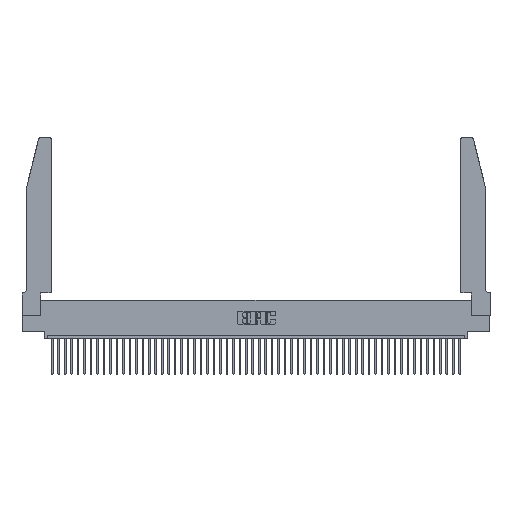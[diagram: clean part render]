
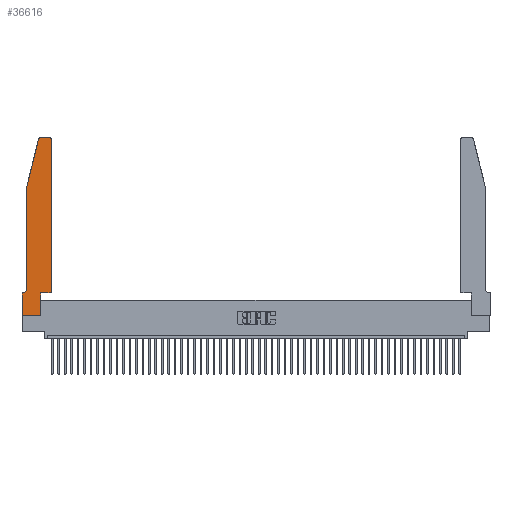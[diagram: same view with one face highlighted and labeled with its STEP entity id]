
A CAD part, top view. The second image highlights one B-rep face of the part: STEP entity #36616.
In plain terms, the highlighted planar face has unit normal (0, 0, 1).
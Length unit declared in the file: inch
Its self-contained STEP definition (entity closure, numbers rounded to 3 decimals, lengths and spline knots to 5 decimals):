
#546 = VECTOR ( 'NONE', #32866, 39.37008 ) ;
#928 = DIRECTION ( 'NONE',  ( 1., 0., 0. ) ) ;
#1456 = ORIENTED_EDGE ( 'NONE', *, *, #26415, .T. ) ;
#2558 = VERTEX_POINT ( 'NONE', #14440 ) ;
#3443 = VERTEX_POINT ( 'NONE', #38005 ) ;
#3659 = VERTEX_POINT ( 'NONE', #14389 ) ;
#3855 = EDGE_CURVE ( 'NONE', #31584, #44310, #7764, .T. ) ;
#4008 = VERTEX_POINT ( 'NONE', #12198 ) ;
#4090 = DIRECTION ( 'NONE',  ( 1., 0., 0. ) ) ;
#5815 = CARTESIAN_POINT ( 'NONE',  ( 0.2865, 0.35, 0.37 ) ) ;
#6371 = DIRECTION ( 'NONE',  ( 0., 0., 1. ) ) ;
#7077 = VERTEX_POINT ( 'NONE', #15256 ) ;
#7407 = VERTEX_POINT ( 'NONE', #23705 ) ;
#7764 = LINE ( 'NONE', #5815, #47663 ) ;
#8116 = EDGE_CURVE ( 'NONE', #3443, #46288, #13813, .T. ) ;
#8571 = CARTESIAN_POINT ( 'NONE',  ( 0.0755, 2., 0.37 ) ) ;
#8710 = DIRECTION ( 'NONE',  ( -1., 0., 0. ) ) ;
#8753 = PLANE ( 'NONE',  #46089 ) ;
#8880 = CARTESIAN_POINT ( 'NONE',  ( 0.0755, 0.35, 0.37 ) ) ;
#9929 = CARTESIAN_POINT ( 'NONE',  ( 0.284, 2.72, 0.37 ) ) ;
#10251 = AXIS2_PLACEMENT_3D ( 'NONE', #9929, #6371, #37412 ) ;
#11137 = EDGE_CURVE ( 'NONE', #2558, #7077, #17133, .T. ) ;
#11425 = EDGE_CURVE ( 'NONE', #7407, #22206, #19561, .T. ) ;
#12198 = CARTESIAN_POINT ( 'NONE',  ( 0.0055, 0.35, 0.37 ) ) ;
#12435 = CARTESIAN_POINT ( 'NONE',  ( 0., 0.35, 0.37 ) ) ;
#13041 = ORIENTED_EDGE ( 'NONE', *, *, #32756, .T. ) ;
#13813 = LINE ( 'NONE', #17291, #546 ) ;
#14202 = LINE ( 'NONE', #15179, #27502 ) ;
#14389 = CARTESIAN_POINT ( 'NONE',  ( 0.0755, 0.42, 0.37 ) ) ;
#14440 = CARTESIAN_POINT ( 'NONE',  ( 0.284, 2.75, 0.37 ) ) ;
#14837 = VECTOR ( 'NONE', #25007, 39.37008 ) ;
#14989 = LINE ( 'NONE', #8880, #25309 ) ;
#15179 = CARTESIAN_POINT ( 'NONE',  ( 0., 0., 0.37 ) ) ;
#15256 = CARTESIAN_POINT ( 'NONE',  ( 0.25487, 2.72718, 0.37 ) ) ;
#15302 = EDGE_CURVE ( 'NONE', #37800, #7407, #28854, .T. ) ;
#15967 = EDGE_CURVE ( 'NONE', #22206, #2558, #49955, .T. ) ;
#16433 = ORIENTED_EDGE ( 'NONE', *, *, #26917, .T. ) ;
#17133 = CIRCLE ( 'NONE', #10251, 0.03 ) ;
#17291 = CARTESIAN_POINT ( 'NONE',  ( 0., 0., 0.37 ) ) ;
#17758 = DIRECTION ( 'NONE',  ( 0., 1., 0. ) ) ;
#17773 = DIRECTION ( 'NONE',  ( 0., 1., 0. ) ) ;
#17872 = CARTESIAN_POINT ( 'NONE',  ( 0.2605, 2.75, 0.37 ) ) ;
#17987 = VECTOR ( 'NONE', #27104, 39.37008 ) ;
#19561 = CIRCLE ( 'NONE', #27385, 0.03 ) ;
#20211 = DIRECTION ( 'NONE',  ( 0., 0., 1. ) ) ;
#21271 = ORIENTED_EDGE ( 'NONE', *, *, #8116, .T. ) ;
#22206 = VERTEX_POINT ( 'NONE', #24424 ) ;
#22641 = DIRECTION ( 'NONE',  ( 1., 0., 0. ) ) ;
#22766 = ORIENTED_EDGE ( 'NONE', *, *, #11137, .T. ) ;
#23705 = CARTESIAN_POINT ( 'NONE',  ( 0.4505, 2.72, 0.37 ) ) ;
#24014 = VERTEX_POINT ( 'NONE', #43203 ) ;
#24424 = CARTESIAN_POINT ( 'NONE',  ( 0.4205, 2.75, 0.37 ) ) ;
#25007 = DIRECTION ( 'NONE',  ( -0.239, -0.971, 0. ) ) ;
#25309 = VECTOR ( 'NONE', #8710, 39.37008 ) ;
#26415 = EDGE_CURVE ( 'NONE', #4008, #3443, #14989, .T. ) ;
#26917 = EDGE_CURVE ( 'NONE', #24014, #3659, #30052, .T. ) ;
#27104 = DIRECTION ( 'NONE',  ( 0., -1., 0. ) ) ;
#27198 = CARTESIAN_POINT ( 'NONE',  ( 0.4205, 2.72, 0.37 ) ) ;
#27385 = AXIS2_PLACEMENT_3D ( 'NONE', #27198, #47868, #4090 ) ;
#27502 = VECTOR ( 'NONE', #22641, 39.37008 ) ;
#27690 = CARTESIAN_POINT ( 'NONE',  ( 0., 0., 0.37 ) ) ;
#27710 = ORIENTED_EDGE ( 'NONE', *, *, #15302, .T. ) ;
#28151 = DIRECTION ( 'NONE',  ( 0., 0., -1. ) ) ;
#28197 = EDGE_CURVE ( 'NONE', #3659, #4008, #41419, .T. ) ;
#28606 = ORIENTED_EDGE ( 'NONE', *, *, #28814, .T. ) ;
#28814 = EDGE_CURVE ( 'NONE', #44310, #37800, #40787, .T. ) ;
#28841 = ORIENTED_EDGE ( 'NONE', *, *, #28197, .T. ) ;
#28854 = LINE ( 'NONE', #48570, #44589 ) ;
#28858 = CARTESIAN_POINT ( 'NONE',  ( 0.4505, 0.35, 0.37 ) ) ;
#29284 = VECTOR ( 'NONE', #47081, 39.37008 ) ;
#30052 = LINE ( 'NONE', #8571, #17987 ) ;
#31584 = VERTEX_POINT ( 'NONE', #42080 ) ;
#31623 = CARTESIAN_POINT ( 'NONE',  ( 0.0755, 2., 0.37 ) ) ;
#32061 = DIRECTION ( 'NONE',  ( -1., 0., 0. ) ) ;
#32756 = EDGE_CURVE ( 'NONE', #7077, #24014, #42079, .T. ) ;
#32866 = DIRECTION ( 'NONE',  ( 0., -1., 0. ) ) ;
#33287 = DIRECTION ( 'NONE',  ( -1., 0., 0. ) ) ;
#33445 = EDGE_LOOP ( 'NONE', ( #35763, #22766, #13041, #16433, #28841, #1456, #21271, #37158, #45116, #28606, #27710, #37364 ) ) ;
#35763 = ORIENTED_EDGE ( 'NONE', *, *, #15967, .T. ) ;
#36616 = ADVANCED_FACE ( 'NONE', ( #47873 ), #8753, .T. ) ;
#37158 = ORIENTED_EDGE ( 'NONE', *, *, #42942, .T. ) ;
#37364 = ORIENTED_EDGE ( 'NONE', *, *, #11425, .T. ) ;
#37412 = DIRECTION ( 'NONE',  ( 1., 0., 0. ) ) ;
#37681 = AXIS2_PLACEMENT_3D ( 'NONE', #47123, #28151, #32061 ) ;
#37800 = VERTEX_POINT ( 'NONE', #28858 ) ;
#38005 = CARTESIAN_POINT ( 'NONE',  ( 0., 0.35, 0.37 ) ) ;
#40787 = LINE ( 'NONE', #43188, #29284 ) ;
#41419 = CIRCLE ( 'NONE', #37681, 0.07 ) ;
#42079 = LINE ( 'NONE', #31623, #14837 ) ;
#42080 = CARTESIAN_POINT ( 'NONE',  ( 0.2865, 0., 0.37 ) ) ;
#42942 = EDGE_CURVE ( 'NONE', #46288, #31584, #14202, .T. ) ;
#43188 = CARTESIAN_POINT ( 'NONE',  ( 0.4505, 0.35, 0.37 ) ) ;
#43203 = CARTESIAN_POINT ( 'NONE',  ( 0.0755, 2., 0.37 ) ) ;
#44310 = VERTEX_POINT ( 'NONE', #45110 ) ;
#44589 = VECTOR ( 'NONE', #17773, 39.37008 ) ;
#45110 = CARTESIAN_POINT ( 'NONE',  ( 0.2865, 0.35, 0.37 ) ) ;
#45116 = ORIENTED_EDGE ( 'NONE', *, *, #3855, .T. ) ;
#46089 = AXIS2_PLACEMENT_3D ( 'NONE', #12435, #20211, #928 ) ;
#46288 = VERTEX_POINT ( 'NONE', #27690 ) ;
#46340 = VECTOR ( 'NONE', #33287, 39.37008 ) ;
#47081 = DIRECTION ( 'NONE',  ( 1., 0., 0. ) ) ;
#47123 = CARTESIAN_POINT ( 'NONE',  ( 0.0055, 0.42, 0.37 ) ) ;
#47663 = VECTOR ( 'NONE', #17758, 39.37008 ) ;
#47868 = DIRECTION ( 'NONE',  ( 0., 0., 1. ) ) ;
#47873 = FACE_OUTER_BOUND ( 'NONE', #33445, .T. ) ;
#48570 = CARTESIAN_POINT ( 'NONE',  ( 0.4505, 0.35, 0.37 ) ) ;
#49955 = LINE ( 'NONE', #17872, #46340 ) ;
